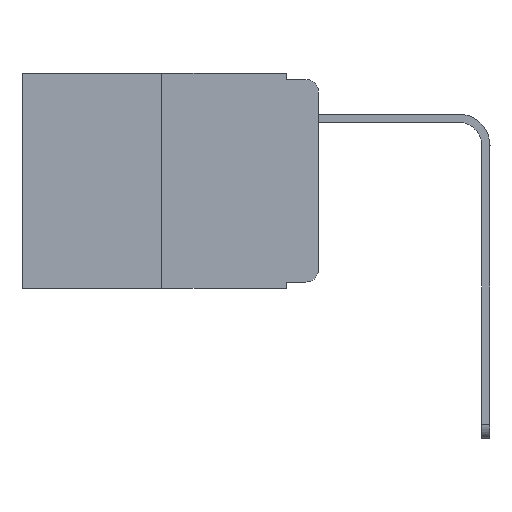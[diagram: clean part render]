
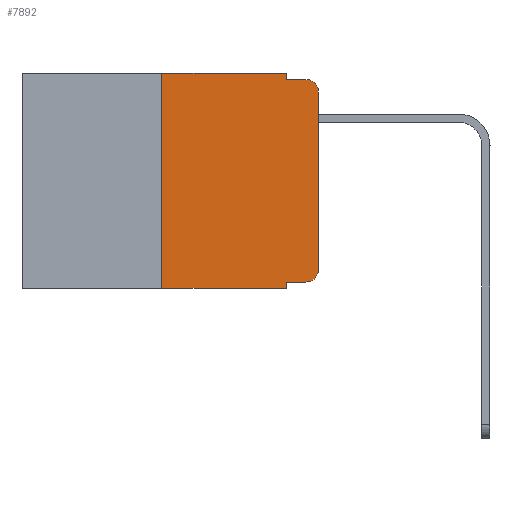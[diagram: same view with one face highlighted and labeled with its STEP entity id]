
A CAD part, left-side view. The second image highlights one B-rep face of the part: STEP entity #7892.
In plain terms, the highlighted planar face has unit normal (-1, 0, 0).
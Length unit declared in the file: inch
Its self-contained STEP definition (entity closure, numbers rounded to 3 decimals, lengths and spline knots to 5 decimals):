
#908 = DIRECTION ( 'NONE',  ( 0., 0., -1. ) ) ;
#992 = EDGE_CURVE ( 'NONE', #11262, #3764, #16524, .T. ) ;
#1127 = EDGE_CURVE ( 'NONE', #13854, #15921, #6425, .T. ) ;
#1260 = LINE ( 'NONE', #13716, #16181 ) ;
#1436 = VERTEX_POINT ( 'NONE', #6934 ) ;
#1449 = CARTESIAN_POINT ( 'NONE',  ( 0., 0.051, -0.01 ) ) ;
#1632 = VERTEX_POINT ( 'NONE', #16132 ) ;
#1669 = CARTESIAN_POINT ( 'NONE',  ( 0., 0.473, -0.343 ) ) ;
#2071 = DIRECTION ( 'NONE',  ( 0., 0., 1. ) ) ;
#2128 = CARTESIAN_POINT ( 'NONE',  ( 0., 0., 0. ) ) ;
#2220 = LINE ( 'NONE', #7556, #10483 ) ;
#2243 = LINE ( 'NONE', #7146, #9497 ) ;
#2337 = VECTOR ( 'NONE', #9204, 39.37008 ) ;
#2776 = CIRCLE ( 'NONE', #5911, 0.02 ) ;
#2846 = LINE ( 'NONE', #1669, #13121 ) ;
#3247 = CARTESIAN_POINT ( 'NONE',  ( 0., 0.051, 0. ) ) ;
#3733 = CARTESIAN_POINT ( 'NONE',  ( 0., 0.02, -0.03 ) ) ;
#3764 = VERTEX_POINT ( 'NONE', #7591 ) ;
#3932 = ORIENTED_EDGE ( 'NONE', *, *, #12072, .F. ) ;
#3963 = VECTOR ( 'NONE', #4697, 39.37008 ) ;
#4014 = EDGE_CURVE ( 'NONE', #1436, #11262, #5743, .T. ) ;
#4068 = FACE_OUTER_BOUND ( 'NONE', #8546, .T. ) ;
#4227 = CARTESIAN_POINT ( 'NONE',  ( 0., 0.25, 0. ) ) ;
#4492 = VERTEX_POINT ( 'NONE', #5188 ) ;
#4595 = CARTESIAN_POINT ( 'NONE',  ( 0., 0.051, 0. ) ) ;
#4697 = DIRECTION ( 'NONE',  ( 0., 0., -1. ) ) ;
#5188 = CARTESIAN_POINT ( 'NONE',  ( 0., 0.051, -0.343 ) ) ;
#5553 = DIRECTION ( 'NONE',  ( 0., 0., -1. ) ) ;
#5743 = LINE ( 'NONE', #10469, #2337 ) ;
#5911 = AXIS2_PLACEMENT_3D ( 'NONE', #3733, #6117, #10088 ) ;
#6029 = VECTOR ( 'NONE', #7019, 39.37008 ) ;
#6117 = DIRECTION ( 'NONE',  ( -1., 0., 0. ) ) ;
#6425 = LINE ( 'NONE', #12077, #6029 ) ;
#6434 = ORIENTED_EDGE ( 'NONE', *, *, #13782, .F. ) ;
#6638 = ORIENTED_EDGE ( 'NONE', *, *, #7789, .T. ) ;
#6666 = ORIENTED_EDGE ( 'NONE', *, *, #8656, .T. ) ;
#6934 = CARTESIAN_POINT ( 'NONE',  ( 0., 0.051, -0.333 ) ) ;
#7019 = DIRECTION ( 'NONE',  ( 0., 0., -1. ) ) ;
#7146 = CARTESIAN_POINT ( 'NONE',  ( 0., 0.473, 0. ) ) ;
#7245 = LINE ( 'NONE', #2128, #11697 ) ;
#7531 = VERTEX_POINT ( 'NONE', #14661 ) ;
#7556 = CARTESIAN_POINT ( 'NONE',  ( 0., 0.051, -0.01 ) ) ;
#7591 = CARTESIAN_POINT ( 'NONE',  ( 0., 0., -0.313 ) ) ;
#7789 = EDGE_CURVE ( 'NONE', #1632, #4492, #2846, .T. ) ;
#7892 = ADVANCED_FACE ( 'NONE', ( #4068 ), #8490, .F. ) ;
#8159 = DIRECTION ( 'NONE',  ( 0., -1., 0. ) ) ;
#8383 = CARTESIAN_POINT ( 'NONE',  ( 0., 0., -0.03 ) ) ;
#8490 = PLANE ( 'NONE',  #16265 ) ;
#8546 = EDGE_LOOP ( 'NONE', ( #6666, #15159, #14563, #12500, #6434, #3932, #6638, #13622, #15353, #12088 ) ) ;
#8656 = EDGE_CURVE ( 'NONE', #3764, #13862, #7245, .T. ) ;
#9204 = DIRECTION ( 'NONE',  ( 0., -1., 0. ) ) ;
#9225 = CARTESIAN_POINT ( 'NONE',  ( 0., 0.02, -0.333 ) ) ;
#9497 = VECTOR ( 'NONE', #8159, 39.37008 ) ;
#10042 = EDGE_CURVE ( 'NONE', #13862, #7531, #2776, .T. ) ;
#10088 = DIRECTION ( 'NONE',  ( 0., 0., -1. ) ) ;
#10469 = CARTESIAN_POINT ( 'NONE',  ( 0., 0.051, -0.333 ) ) ;
#10483 = VECTOR ( 'NONE', #16596, 39.37008 ) ;
#11229 = VERTEX_POINT ( 'NONE', #4227 ) ;
#11262 = VERTEX_POINT ( 'NONE', #9225 ) ;
#11697 = VECTOR ( 'NONE', #2071, 39.37008 ) ;
#12072 = EDGE_CURVE ( 'NONE', #1632, #11229, #1260, .T. ) ;
#12077 = CARTESIAN_POINT ( 'NONE',  ( 0., 0.051, 0. ) ) ;
#12088 = ORIENTED_EDGE ( 'NONE', *, *, #992, .T. ) ;
#12500 = ORIENTED_EDGE ( 'NONE', *, *, #1127, .F. ) ;
#12580 = CARTESIAN_POINT ( 'NONE',  ( 0., 0.473, 0. ) ) ;
#13121 = VECTOR ( 'NONE', #13171, 39.37008 ) ;
#13171 = DIRECTION ( 'NONE',  ( 0., -1., 0. ) ) ;
#13622 = ORIENTED_EDGE ( 'NONE', *, *, #16681, .F. ) ;
#13716 = CARTESIAN_POINT ( 'NONE',  ( 0., 0.25, 0. ) ) ;
#13782 = EDGE_CURVE ( 'NONE', #11229, #13854, #2243, .T. ) ;
#13798 = AXIS2_PLACEMENT_3D ( 'NONE', #15873, #15926, #5553 ) ;
#13805 = DIRECTION ( 'NONE',  ( 1., 0., 0. ) ) ;
#13854 = VERTEX_POINT ( 'NONE', #4595 ) ;
#13862 = VERTEX_POINT ( 'NONE', #8383 ) ;
#14210 = LINE ( 'NONE', #3247, #3963 ) ;
#14563 = ORIENTED_EDGE ( 'NONE', *, *, #14821, .F. ) ;
#14661 = CARTESIAN_POINT ( 'NONE',  ( 0., 0.02, -0.01 ) ) ;
#14821 = EDGE_CURVE ( 'NONE', #15921, #7531, #2220, .T. ) ;
#15013 = DIRECTION ( 'NONE',  ( 0., 0., 1. ) ) ;
#15159 = ORIENTED_EDGE ( 'NONE', *, *, #10042, .T. ) ;
#15353 = ORIENTED_EDGE ( 'NONE', *, *, #4014, .T. ) ;
#15873 = CARTESIAN_POINT ( 'NONE',  ( 0., 0.02, -0.313 ) ) ;
#15921 = VERTEX_POINT ( 'NONE', #1449 ) ;
#15926 = DIRECTION ( 'NONE',  ( -1., 0., 0. ) ) ;
#16132 = CARTESIAN_POINT ( 'NONE',  ( 0., 0.25, -0.343 ) ) ;
#16181 = VECTOR ( 'NONE', #15013, 39.37008 ) ;
#16265 = AXIS2_PLACEMENT_3D ( 'NONE', #12580, #13805, #908 ) ;
#16524 = CIRCLE ( 'NONE', #13798, 0.02 ) ;
#16596 = DIRECTION ( 'NONE',  ( 0., -1., 0. ) ) ;
#16681 = EDGE_CURVE ( 'NONE', #1436, #4492, #14210, .T. ) ;
